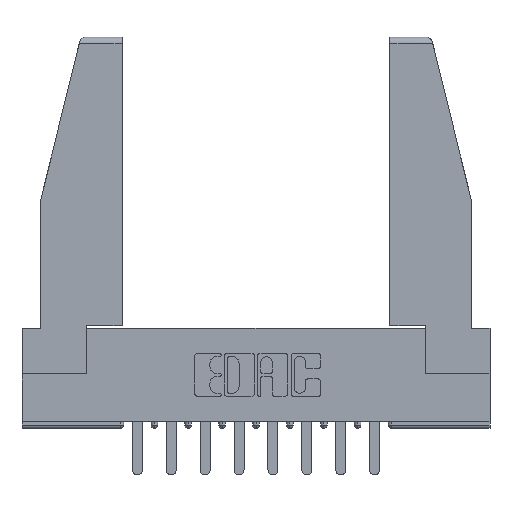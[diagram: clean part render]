
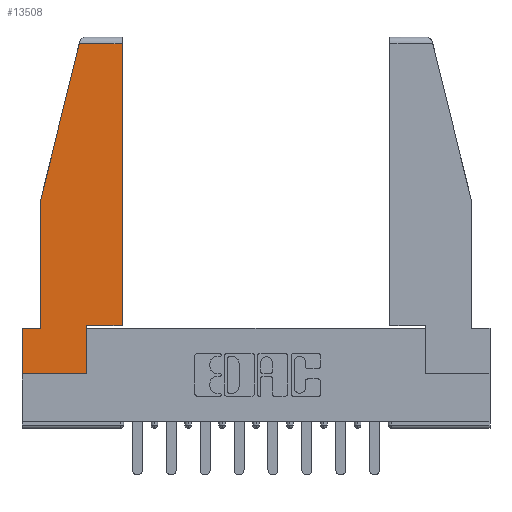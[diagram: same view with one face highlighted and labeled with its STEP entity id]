
A CAD part, top view. The second image highlights one B-rep face of the part: STEP entity #13508.
In plain terms, the highlighted planar face has unit normal (0, 0, 1).
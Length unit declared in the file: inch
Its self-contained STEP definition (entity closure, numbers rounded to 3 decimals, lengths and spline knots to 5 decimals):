
#48 = DIRECTION ( 'NONE',  ( 1., 0., 0. ) ) ;
#373 = CARTESIAN_POINT ( 'NONE',  ( 0.297, 0.223, 0. ) ) ;
#385 = EDGE_CURVE ( 'NONE', #13802, #4459, #5907, .T. ) ;
#440 = CARTESIAN_POINT ( 'NONE',  ( 0.2636, 1.52, 0. ) ) ;
#482 = DIRECTION ( 'NONE',  ( -0.239, -0.971, 0. ) ) ;
#833 = VECTOR ( 'NONE', #2340, 39.37008 ) ;
#849 = ORIENTED_EDGE ( 'NONE', *, *, #9400, .T. ) ;
#1249 = EDGE_CURVE ( 'NONE', #3818, #4982, #6905, .T. ) ;
#1284 = CARTESIAN_POINT ( 'NONE',  ( 0.271, 1.55, 0. ) ) ;
#1454 = EDGE_CURVE ( 'NONE', #10829, #3818, #7076, .T. ) ;
#1875 = FACE_OUTER_BOUND ( 'NONE', #8025, .T. ) ;
#2340 = DIRECTION ( 'NONE',  ( -1., 0., 0. ) ) ;
#2482 = CARTESIAN_POINT ( 'NONE',  ( 0.086, 0.8, 0. ) ) ;
#2684 = DIRECTION ( 'NONE',  ( 0., 1., 0. ) ) ;
#2866 = DIRECTION ( 'NONE',  ( 0., 1., 0. ) ) ;
#3119 = PLANE ( 'NONE',  #5421 ) ;
#3194 = DIRECTION ( 'NONE',  ( 0., -1., 0. ) ) ;
#3423 = CARTESIAN_POINT ( 'NONE',  ( 0., 0.21, 0. ) ) ;
#3559 = CARTESIAN_POINT ( 'NONE',  ( 0.086, 0.21, 0. ) ) ;
#3569 = VECTOR ( 'NONE', #48, 39.37008 ) ;
#3818 = VERTEX_POINT ( 'NONE', #8128 ) ;
#4049 = ORIENTED_EDGE ( 'NONE', *, *, #4364, .T. ) ;
#4120 = CARTESIAN_POINT ( 'NONE',  ( 0., 0., 0. ) ) ;
#4151 = VECTOR ( 'NONE', #2684, 39.37008 ) ;
#4252 = DIRECTION ( 'NONE',  ( 1., 0., 0. ) ) ;
#4364 = EDGE_CURVE ( 'NONE', #4982, #13802, #7690, .T. ) ;
#4437 = ORIENTED_EDGE ( 'NONE', *, *, #10484, .T. ) ;
#4459 = VERTEX_POINT ( 'NONE', #3559 ) ;
#4748 = EDGE_CURVE ( 'NONE', #13594, #7363, #8029, .T. ) ;
#4982 = VERTEX_POINT ( 'NONE', #440 ) ;
#5107 = VECTOR ( 'NONE', #6375, 39.37008 ) ;
#5269 = DIRECTION ( 'NONE',  ( 0., -1., 0. ) ) ;
#5421 = AXIS2_PLACEMENT_3D ( 'NONE', #6216, #10840, #4252 ) ;
#5476 = EDGE_CURVE ( 'NONE', #4459, #11260, #13251, .T. ) ;
#5907 = LINE ( 'NONE', #14250, #11368 ) ;
#6058 = VECTOR ( 'NONE', #2866, 39.37008 ) ;
#6143 = CARTESIAN_POINT ( 'NONE',  ( 0., 1.52, 0. ) ) ;
#6190 = ORIENTED_EDGE ( 'NONE', *, *, #1454, .T. ) ;
#6216 = CARTESIAN_POINT ( 'NONE',  ( 0., 0., 0. ) ) ;
#6375 = DIRECTION ( 'NONE',  ( 1., 0., 0. ) ) ;
#6788 = EDGE_CURVE ( 'NONE', #7363, #8503, #11505, .T. ) ;
#6874 = ORIENTED_EDGE ( 'NONE', *, *, #6788, .T. ) ;
#6905 = LINE ( 'NONE', #6143, #9533 ) ;
#7076 = LINE ( 'NONE', #10683, #4151 ) ;
#7157 = CARTESIAN_POINT ( 'NONE',  ( 0.297, 0., 0. ) ) ;
#7363 = VERTEX_POINT ( 'NONE', #7157 ) ;
#7690 = LINE ( 'NONE', #1284, #10331 ) ;
#7717 = DIRECTION ( 'NONE',  ( -1., 0., 0. ) ) ;
#8025 = EDGE_LOOP ( 'NONE', ( #6190, #9687, #4049, #8836, #14225, #4437, #12473, #6874, #849 ) ) ;
#8029 = LINE ( 'NONE', #4120, #5107 ) ;
#8128 = CARTESIAN_POINT ( 'NONE',  ( 0.461, 1.52, 0. ) ) ;
#8392 = CARTESIAN_POINT ( 'NONE',  ( 0.297, 0., 0. ) ) ;
#8503 = VERTEX_POINT ( 'NONE', #373 ) ;
#8836 = ORIENTED_EDGE ( 'NONE', *, *, #385, .T. ) ;
#9400 = EDGE_CURVE ( 'NONE', #8503, #10829, #9811, .T. ) ;
#9533 = VECTOR ( 'NONE', #7717, 39.37008 ) ;
#9687 = ORIENTED_EDGE ( 'NONE', *, *, #1249, .T. ) ;
#9811 = LINE ( 'NONE', #10083, #3569 ) ;
#10083 = CARTESIAN_POINT ( 'NONE',  ( 0.297, 0.223, 0. ) ) ;
#10176 = CARTESIAN_POINT ( 'NONE',  ( 0., 0.21, 0. ) ) ;
#10314 = VECTOR ( 'NONE', #3194, 39.37008 ) ;
#10331 = VECTOR ( 'NONE', #482, 39.37008 ) ;
#10484 = EDGE_CURVE ( 'NONE', #11260, #13594, #13097, .T. ) ;
#10683 = CARTESIAN_POINT ( 'NONE',  ( 0.461, 0.223, 0. ) ) ;
#10829 = VERTEX_POINT ( 'NONE', #11400 ) ;
#10840 = DIRECTION ( 'NONE',  ( 0., 0., 1. ) ) ;
#11260 = VERTEX_POINT ( 'NONE', #10176 ) ;
#11368 = VECTOR ( 'NONE', #5269, 39.37008 ) ;
#11400 = CARTESIAN_POINT ( 'NONE',  ( 0.461, 0.223, 0. ) ) ;
#11505 = LINE ( 'NONE', #8392, #6058 ) ;
#12473 = ORIENTED_EDGE ( 'NONE', *, *, #4748, .T. ) ;
#12997 = CARTESIAN_POINT ( 'NONE',  ( 0., 0.21, 0. ) ) ;
#13097 = LINE ( 'NONE', #12997, #10314 ) ;
#13251 = LINE ( 'NONE', #3423, #833 ) ;
#13508 = ADVANCED_FACE ( 'NONE', ( #1875 ), #3119, .T. ) ;
#13594 = VERTEX_POINT ( 'NONE', #14191 ) ;
#13802 = VERTEX_POINT ( 'NONE', #2482 ) ;
#14191 = CARTESIAN_POINT ( 'NONE',  ( 0., 0., 0. ) ) ;
#14225 = ORIENTED_EDGE ( 'NONE', *, *, #5476, .T. ) ;
#14250 = CARTESIAN_POINT ( 'NONE',  ( 0.086, 0.8, 0. ) ) ;
